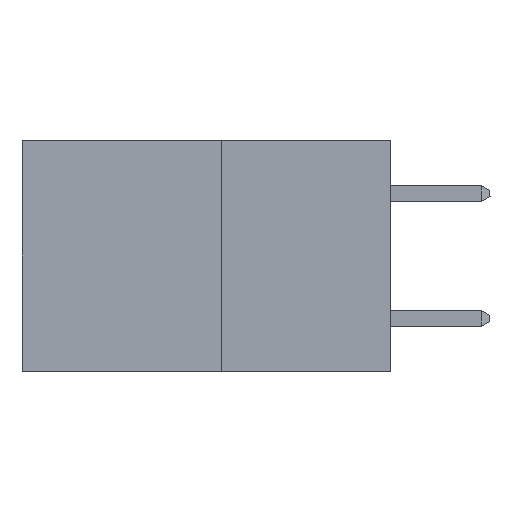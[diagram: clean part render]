
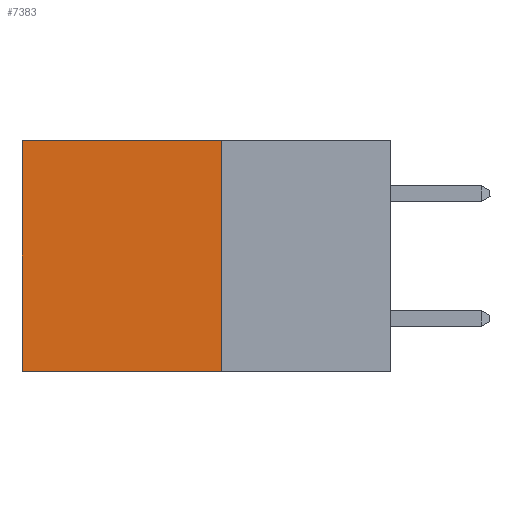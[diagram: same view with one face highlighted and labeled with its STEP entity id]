
A CAD part, left-side view. The second image highlights one B-rep face of the part: STEP entity #7383.
In plain terms, the highlighted planar face has unit normal (-1, 0, 0).
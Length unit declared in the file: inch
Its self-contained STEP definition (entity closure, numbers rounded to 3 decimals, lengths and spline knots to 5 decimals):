
#412 = CARTESIAN_POINT ( 'NONE',  ( 0.277, 0.27, 0. ) ) ;
#733 = DIRECTION ( 'NONE',  ( 0., 0., -1. ) ) ;
#873 = CARTESIAN_POINT ( 'NONE',  ( 0.277, 0.27, -0.37 ) ) ;
#1920 = EDGE_CURVE ( 'NONE', #6642, #14893, #16882, .T. ) ;
#2224 = DIRECTION ( 'NONE',  ( 0., 0., -1. ) ) ;
#2470 = EDGE_LOOP ( 'NONE', ( #12183, #3359, #7938, #7540 ) ) ;
#3359 = ORIENTED_EDGE ( 'NONE', *, *, #15952, .F. ) ;
#3854 = VERTEX_POINT ( 'NONE', #14875 ) ;
#5593 = AXIS2_PLACEMENT_3D ( 'NONE', #873, #10203, #2224 ) ;
#5671 = LINE ( 'NONE', #12763, #9200 ) ;
#6629 = VECTOR ( 'NONE', #13456, 39.37008 ) ;
#6642 = VERTEX_POINT ( 'NONE', #412 ) ;
#7383 = ADVANCED_FACE ( 'NONE', ( #15321 ), #16891, .F. ) ;
#7540 = ORIENTED_EDGE ( 'NONE', *, *, #1920, .T. ) ;
#7938 = ORIENTED_EDGE ( 'NONE', *, *, #8039, .F. ) ;
#8039 = EDGE_CURVE ( 'NONE', #6642, #8217, #5671, .T. ) ;
#8217 = VERTEX_POINT ( 'NONE', #13113 ) ;
#8350 = VECTOR ( 'NONE', #11431, 39.37008 ) ;
#9200 = VECTOR ( 'NONE', #733, 39.37008 ) ;
#9648 = DIRECTION ( 'NONE',  ( 0., 1., 0. ) ) ;
#10203 = DIRECTION ( 'NONE',  ( 1., 0., 0. ) ) ;
#11431 = DIRECTION ( 'NONE',  ( 0., 0., -1. ) ) ;
#11895 = LINE ( 'NONE', #16773, #8350 ) ;
#12183 = ORIENTED_EDGE ( 'NONE', *, *, #15566, .T. ) ;
#12292 = CARTESIAN_POINT ( 'NONE',  ( 0.277, 0.27, 0. ) ) ;
#12763 = CARTESIAN_POINT ( 'NONE',  ( 0.277, 0.27, -0.37 ) ) ;
#13113 = CARTESIAN_POINT ( 'NONE',  ( 0.277, 0.27, -0.37 ) ) ;
#13155 = VECTOR ( 'NONE', #9648, 39.37008 ) ;
#13456 = DIRECTION ( 'NONE',  ( 0., 1., 0. ) ) ;
#14875 = CARTESIAN_POINT ( 'NONE',  ( 0.277, 0.59, -0.37 ) ) ;
#14893 = VERTEX_POINT ( 'NONE', #16794 ) ;
#14994 = CARTESIAN_POINT ( 'NONE',  ( 0.277, 0.27, -0.37 ) ) ;
#15321 = FACE_OUTER_BOUND ( 'NONE', #2470, .T. ) ;
#15566 = EDGE_CURVE ( 'NONE', #14893, #3854, #11895, .T. ) ;
#15952 = EDGE_CURVE ( 'NONE', #8217, #3854, #16719, .T. ) ;
#16719 = LINE ( 'NONE', #14994, #13155 ) ;
#16773 = CARTESIAN_POINT ( 'NONE',  ( 0.277, 0.59, -0.37 ) ) ;
#16794 = CARTESIAN_POINT ( 'NONE',  ( 0.277, 0.59, 0. ) ) ;
#16882 = LINE ( 'NONE', #12292, #6629 ) ;
#16891 = PLANE ( 'NONE',  #5593 ) ;
